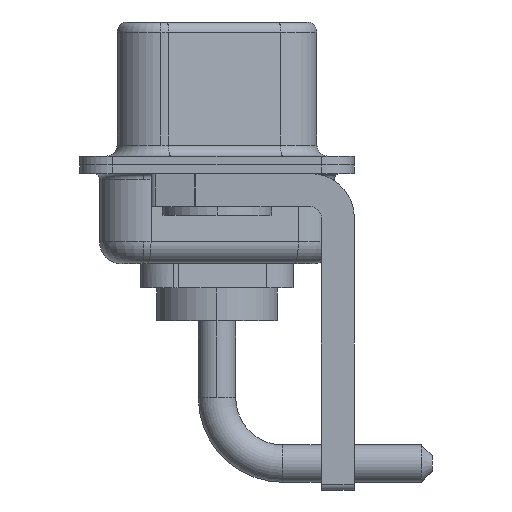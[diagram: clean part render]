
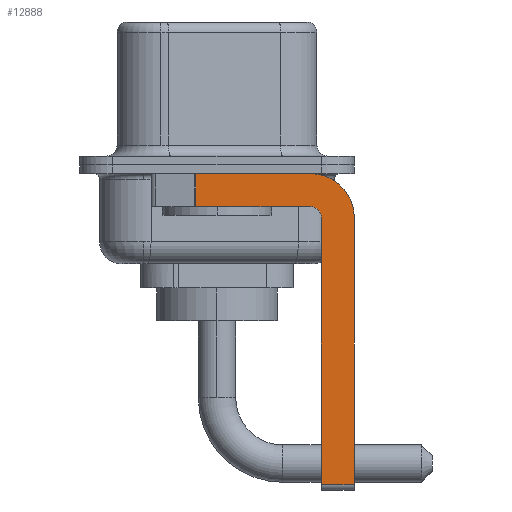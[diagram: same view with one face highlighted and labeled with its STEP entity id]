
A CAD part, left-side view. The second image highlights one B-rep face of the part: STEP entity #12888.
In plain terms, the highlighted planar face has unit normal (-1, 0, 0).
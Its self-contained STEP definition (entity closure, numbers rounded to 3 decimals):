
#495 = LINE ( 'NONE', #6011, #10622 ) ;
#665 = DIRECTION ( 'NONE',  ( 0., 1., 0. ) ) ;
#671 = VERTEX_POINT ( 'NONE', #6139 ) ;
#782 = DIRECTION ( 'NONE',  ( -1., 0., 0. ) ) ;
#1214 = DIRECTION ( 'NONE',  ( 0., 0., -1. ) ) ;
#1412 = EDGE_CURVE ( 'NONE', #8743, #3105, #10285, .T. ) ;
#1427 = CARTESIAN_POINT ( 'NONE',  ( -2.9, -4.25, -14.55 ) ) ;
#1580 = VECTOR ( 'NONE', #4209, 1000. ) ;
#2215 = DIRECTION ( 'NONE',  ( 0., 0., 1. ) ) ;
#2531 = DIRECTION ( 'NONE',  ( 0., 0., 1. ) ) ;
#2777 = ORIENTED_EDGE ( 'NONE', *, *, #7755, .T. ) ;
#3105 = VERTEX_POINT ( 'NONE', #7268 ) ;
#3334 = VERTEX_POINT ( 'NONE', #4489 ) ;
#3750 = DIRECTION ( 'NONE',  ( 0., 0., -1. ) ) ;
#3864 = EDGE_CURVE ( 'NONE', #3105, #671, #495, .T. ) ;
#4024 = AXIS2_PLACEMENT_3D ( 'NONE', #14930, #782, #2215 ) ;
#4192 = EDGE_LOOP ( 'NONE', ( #14376, #2777, #8448, #5825, #6358, #8422, #7578, #14793 ) ) ;
#4202 = EDGE_CURVE ( 'NONE', #15944, #11031, #14377, .T. ) ;
#4209 = DIRECTION ( 'NONE',  ( 0., -1., 0. ) ) ;
#4370 = AXIS2_PLACEMENT_3D ( 'NONE', #10316, #5194, #1214 ) ;
#4489 = CARTESIAN_POINT ( 'NONE',  ( -2.9, 0.978, -0.4 ) ) ;
#4609 = CARTESIAN_POINT ( 'NONE',  ( -2.9, -4.25, -2.4 ) ) ;
#4865 = CARTESIAN_POINT ( 'NONE',  ( -2.9, 0.978, -1.9 ) ) ;
#5194 = DIRECTION ( 'NONE',  ( 1., 0., 0. ) ) ;
#5325 = CARTESIAN_POINT ( 'NONE',  ( -2.9, -4.75, -14.8 ) ) ;
#5339 = EDGE_CURVE ( 'NONE', #3334, #6247, #11141, .T. ) ;
#5825 = ORIENTED_EDGE ( 'NONE', *, *, #1412, .F. ) ;
#5971 = FACE_OUTER_BOUND ( 'NONE', #4192, .T. ) ;
#6011 = CARTESIAN_POINT ( 'NONE',  ( -2.9, -4.25, -1.9 ) ) ;
#6093 = VERTEX_POINT ( 'NONE', #10678 ) ;
#6139 = CARTESIAN_POINT ( 'NONE',  ( -2.9, 0.978, -1.9 ) ) ;
#6247 = VERTEX_POINT ( 'NONE', #12374 ) ;
#6358 = ORIENTED_EDGE ( 'NONE', *, *, #10050, .F. ) ;
#6681 = LINE ( 'NONE', #5325, #11965 ) ;
#7268 = CARTESIAN_POINT ( 'NONE',  ( -2.9, -4.25, -1.9 ) ) ;
#7578 = ORIENTED_EDGE ( 'NONE', *, *, #11865, .F. ) ;
#7631 = DIRECTION ( 'NONE',  ( 0., 0., -1. ) ) ;
#7755 = EDGE_CURVE ( 'NONE', #3334, #671, #11438, .T. ) ;
#8089 = VECTOR ( 'NONE', #3750, 1000. ) ;
#8422 = ORIENTED_EDGE ( 'NONE', *, *, #4202, .T. ) ;
#8448 = ORIENTED_EDGE ( 'NONE', *, *, #3864, .F. ) ;
#8491 = LINE ( 'NONE', #12923, #9798 ) ;
#8743 = VERTEX_POINT ( 'NONE', #11850 ) ;
#9798 = VECTOR ( 'NONE', #7631, 1000. ) ;
#9815 = DIRECTION ( 'NONE',  ( 1., 0., 0. ) ) ;
#10050 = EDGE_CURVE ( 'NONE', #15944, #8743, #6681, .T. ) ;
#10226 = PLANE ( 'NONE',  #4370 ) ;
#10285 = CIRCLE ( 'NONE', #4024, 0.5 ) ;
#10316 = CARTESIAN_POINT ( 'NONE',  ( -2.9, -4.25, -2.4 ) ) ;
#10622 = VECTOR ( 'NONE', #665, 1000. ) ;
#10670 = CIRCLE ( 'NONE', #10952, 2. ) ;
#10678 = CARTESIAN_POINT ( 'NONE',  ( -2.9, -6.25, -2.4 ) ) ;
#10952 = AXIS2_PLACEMENT_3D ( 'NONE', #4609, #9815, #12038 ) ;
#11031 = VERTEX_POINT ( 'NONE', #14709 ) ;
#11141 = LINE ( 'NONE', #11224, #11159 ) ;
#11159 = VECTOR ( 'NONE', #16451, 1000. ) ;
#11224 = CARTESIAN_POINT ( 'NONE',  ( -2.9, 3., -0.4 ) ) ;
#11438 = LINE ( 'NONE', #4865, #8089 ) ;
#11850 = CARTESIAN_POINT ( 'NONE',  ( -2.9, -4.75, -2.4 ) ) ;
#11865 = EDGE_CURVE ( 'NONE', #6093, #11031, #8491, .T. ) ;
#11965 = VECTOR ( 'NONE', #2531, 1000. ) ;
#12038 = DIRECTION ( 'NONE',  ( 0., 0., -1. ) ) ;
#12374 = CARTESIAN_POINT ( 'NONE',  ( -2.9, -4.25, -0.4 ) ) ;
#12888 = ADVANCED_FACE ( 'NONE', ( #5971 ), #10226, .F. ) ;
#12923 = CARTESIAN_POINT ( 'NONE',  ( -2.9, -6.25, -2.4 ) ) ;
#14027 = EDGE_CURVE ( 'NONE', #6247, #6093, #10670, .T. ) ;
#14376 = ORIENTED_EDGE ( 'NONE', *, *, #5339, .F. ) ;
#14377 = LINE ( 'NONE', #1427, #1580 ) ;
#14709 = CARTESIAN_POINT ( 'NONE',  ( -2.9, -6.25, -14.55 ) ) ;
#14793 = ORIENTED_EDGE ( 'NONE', *, *, #14027, .F. ) ;
#14930 = CARTESIAN_POINT ( 'NONE',  ( -2.9, -4.25, -2.4 ) ) ;
#14934 = CARTESIAN_POINT ( 'NONE',  ( -2.9, -4.75, -14.55 ) ) ;
#15944 = VERTEX_POINT ( 'NONE', #14934 ) ;
#16451 = DIRECTION ( 'NONE',  ( 0., -1., 0. ) ) ;
